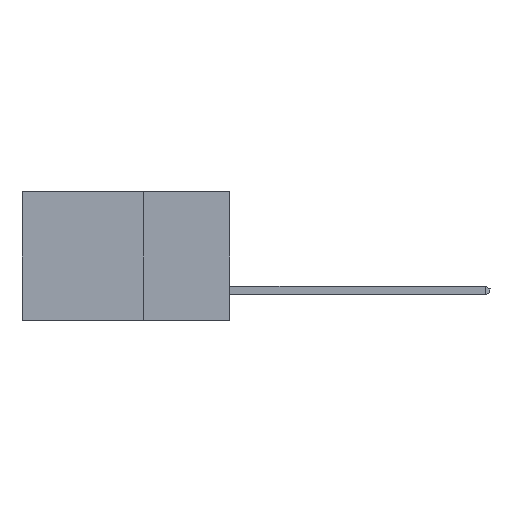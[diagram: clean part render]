
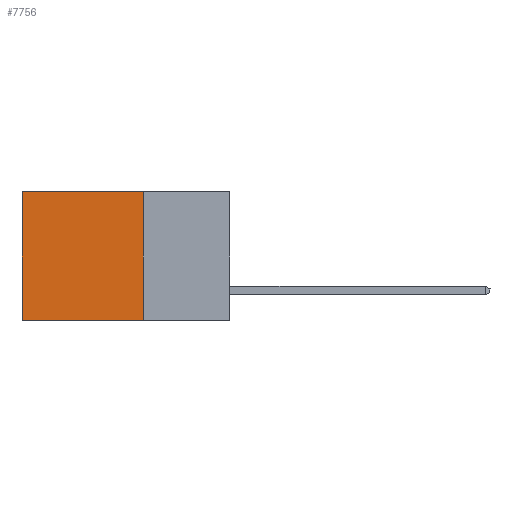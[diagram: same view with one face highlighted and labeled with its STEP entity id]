
A CAD part, left-side view. The second image highlights one B-rep face of the part: STEP entity #7756.
In plain terms, the highlighted planar face has unit normal (-1, 0, 0).
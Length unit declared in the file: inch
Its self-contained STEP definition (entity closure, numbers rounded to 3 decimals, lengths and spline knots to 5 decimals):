
#189 = DIRECTION ( 'NONE',  ( 0., 0., -1. ) ) ;
#1078 = DIRECTION ( 'NONE',  ( 0., 1., 0. ) ) ;
#1123 = ORIENTED_EDGE ( 'NONE', *, *, #12495, .T. ) ;
#1391 = AXIS2_PLACEMENT_3D ( 'NONE', #7479, #2798, #189 ) ;
#1515 = VECTOR ( 'NONE', #11135, 39.37008 ) ;
#1848 = DIRECTION ( 'NONE',  ( 0., 0., -1. ) ) ;
#2209 = PLANE ( 'NONE',  #1391 ) ;
#2798 = DIRECTION ( 'NONE',  ( 1., 0., 0. ) ) ;
#3016 = EDGE_CURVE ( 'NONE', #6302, #7862, #14708, .T. ) ;
#3124 = LINE ( 'NONE', #9676, #1515 ) ;
#3613 = LINE ( 'NONE', #4935, #8651 ) ;
#4835 = LINE ( 'NONE', #15407, #13345 ) ;
#4935 = CARTESIAN_POINT ( 'NONE',  ( 0.2615, 0.6, -0.37 ) ) ;
#5305 = CARTESIAN_POINT ( 'NONE',  ( 0.2615, 0.6, -0.37 ) ) ;
#6302 = VERTEX_POINT ( 'NONE', #8602 ) ;
#6740 = VECTOR ( 'NONE', #1848, 39.37008 ) ;
#6985 = ORIENTED_EDGE ( 'NONE', *, *, #3016, .F. ) ;
#7479 = CARTESIAN_POINT ( 'NONE',  ( 0.2615, 0.25, -0.37 ) ) ;
#7756 = ADVANCED_FACE ( 'NONE', ( #14044 ), #2209, .F. ) ;
#7813 = CARTESIAN_POINT ( 'NONE',  ( 0.2615, 0.25, -0.37 ) ) ;
#7862 = VERTEX_POINT ( 'NONE', #7813 ) ;
#8602 = CARTESIAN_POINT ( 'NONE',  ( 0.2615, 0.25, 0. ) ) ;
#8651 = VECTOR ( 'NONE', #14316, 39.37008 ) ;
#9676 = CARTESIAN_POINT ( 'NONE',  ( 0.2615, 0.25, -0.37 ) ) ;
#10113 = EDGE_CURVE ( 'NONE', #7862, #16931, #3124, .T. ) ;
#10738 = ORIENTED_EDGE ( 'NONE', *, *, #10113, .F. ) ;
#10802 = CARTESIAN_POINT ( 'NONE',  ( 0.2615, 0.6, 0. ) ) ;
#11135 = DIRECTION ( 'NONE',  ( 0., 1., 0. ) ) ;
#11342 = VERTEX_POINT ( 'NONE', #10802 ) ;
#12495 = EDGE_CURVE ( 'NONE', #6302, #11342, #4835, .T. ) ;
#13345 = VECTOR ( 'NONE', #1078, 39.37008 ) ;
#13426 = CARTESIAN_POINT ( 'NONE',  ( 0.2615, 0.25, -0.37 ) ) ;
#14044 = FACE_OUTER_BOUND ( 'NONE', #16856, .T. ) ;
#14262 = EDGE_CURVE ( 'NONE', #11342, #16931, #3613, .T. ) ;
#14316 = DIRECTION ( 'NONE',  ( 0., 0., -1. ) ) ;
#14708 = LINE ( 'NONE', #13426, #6740 ) ;
#15407 = CARTESIAN_POINT ( 'NONE',  ( 0.2615, 0.25, 0. ) ) ;
#15848 = ORIENTED_EDGE ( 'NONE', *, *, #14262, .T. ) ;
#16856 = EDGE_LOOP ( 'NONE', ( #15848, #10738, #6985, #1123 ) ) ;
#16931 = VERTEX_POINT ( 'NONE', #5305 ) ;
